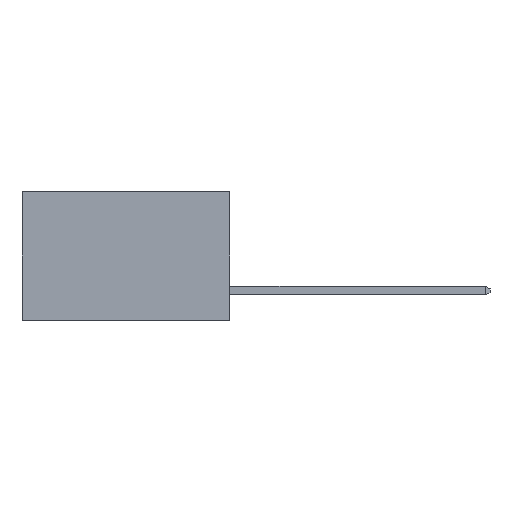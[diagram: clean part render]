
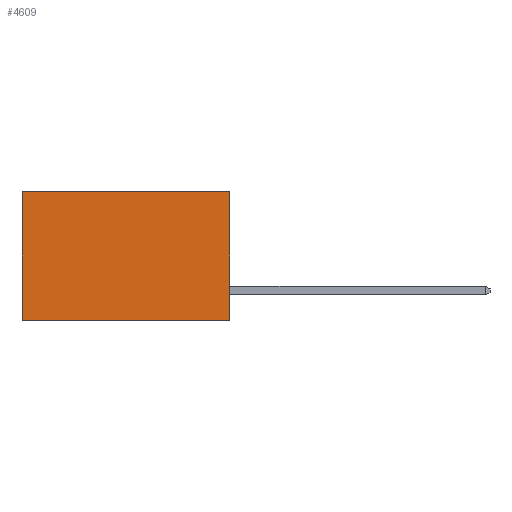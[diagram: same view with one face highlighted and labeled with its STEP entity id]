
A CAD part, left-side view. The second image highlights one B-rep face of the part: STEP entity #4609.
In plain terms, the highlighted planar face has unit normal (-1, 0, 0).
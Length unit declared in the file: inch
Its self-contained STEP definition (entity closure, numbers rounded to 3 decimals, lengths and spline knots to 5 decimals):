
#466 = EDGE_CURVE ( 'NONE', #9389, #4325, #6575, .T. ) ;
#1239 = ORIENTED_EDGE ( 'NONE', *, *, #466, .F. ) ;
#1497 = LINE ( 'NONE', #9819, #12765 ) ;
#2314 = VERTEX_POINT ( 'NONE', #8209 ) ;
#2404 = EDGE_LOOP ( 'NONE', ( #11717, #4160, #1239, #4618 ) ) ;
#3355 = DIRECTION ( 'NONE',  ( 0., 1., 0. ) ) ;
#3420 = VECTOR ( 'NONE', #7634, 39.37008 ) ;
#4160 = ORIENTED_EDGE ( 'NONE', *, *, #4471, .F. ) ;
#4325 = VERTEX_POINT ( 'NONE', #9459 ) ;
#4471 = EDGE_CURVE ( 'NONE', #4325, #5251, #9688, .T. ) ;
#4551 = EDGE_CURVE ( 'NONE', #2314, #5251, #1497, .T. ) ;
#4609 = ADVANCED_FACE ( 'NONE', ( #13540 ), #6230, .F. ) ;
#4618 = ORIENTED_EDGE ( 'NONE', *, *, #4993, .T. ) ;
#4993 = EDGE_CURVE ( 'NONE', #9389, #2314, #11039, .T. ) ;
#5251 = VERTEX_POINT ( 'NONE', #6393 ) ;
#5947 = CARTESIAN_POINT ( 'NONE',  ( 0.298, 0., 0. ) ) ;
#6230 = PLANE ( 'NONE',  #12946 ) ;
#6307 = CARTESIAN_POINT ( 'NONE',  ( 0.298, 0., 0. ) ) ;
#6393 = CARTESIAN_POINT ( 'NONE',  ( 0.298, 0.6, -0.37 ) ) ;
#6411 = CARTESIAN_POINT ( 'NONE',  ( 0.298, 0., 0. ) ) ;
#6575 = LINE ( 'NONE', #5947, #3420 ) ;
#7361 = DIRECTION ( 'NONE',  ( 0., 1., 0. ) ) ;
#7634 = DIRECTION ( 'NONE',  ( 0., 0., -1. ) ) ;
#8209 = CARTESIAN_POINT ( 'NONE',  ( 0.298, 0.6, 0. ) ) ;
#8415 = VECTOR ( 'NONE', #3355, 39.37008 ) ;
#8726 = DIRECTION ( 'NONE',  ( 0., 0., -1. ) ) ;
#8756 = DIRECTION ( 'NONE',  ( 1., 0., 0. ) ) ;
#9385 = VECTOR ( 'NONE', #7361, 39.37008 ) ;
#9389 = VERTEX_POINT ( 'NONE', #9596 ) ;
#9459 = CARTESIAN_POINT ( 'NONE',  ( 0.298, 0., -0.37 ) ) ;
#9596 = CARTESIAN_POINT ( 'NONE',  ( 0.298, 0., 0. ) ) ;
#9688 = LINE ( 'NONE', #9793, #9385 ) ;
#9793 = CARTESIAN_POINT ( 'NONE',  ( 0.298, 0., -0.37 ) ) ;
#9819 = CARTESIAN_POINT ( 'NONE',  ( 0.298, 0.6, 0. ) ) ;
#11039 = LINE ( 'NONE', #6307, #8415 ) ;
#11717 = ORIENTED_EDGE ( 'NONE', *, *, #4551, .T. ) ;
#12720 = DIRECTION ( 'NONE',  ( 0., 0., -1. ) ) ;
#12765 = VECTOR ( 'NONE', #12720, 39.37008 ) ;
#12946 = AXIS2_PLACEMENT_3D ( 'NONE', #6411, #8756, #8726 ) ;
#13540 = FACE_OUTER_BOUND ( 'NONE', #2404, .T. ) ;
